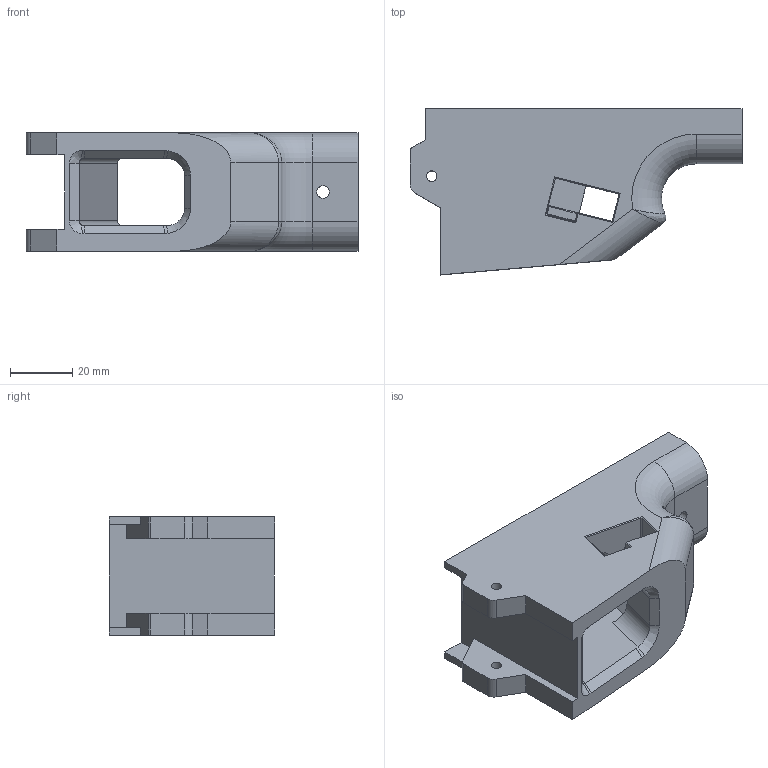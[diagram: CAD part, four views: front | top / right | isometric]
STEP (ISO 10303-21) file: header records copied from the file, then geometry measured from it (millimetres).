
FILE_DESCRIPTION(/* description */ (''),/* implementation_level */ '2;1');
FILE_NAME(/* author */ (''),/* organization */ (''),/* preprocessor_version */ 'ST-DEVELOPER v18.1',/* originating_system */ 'Autodesk Translation Framework v9.3.0.1241',/* authorisation */ '');
FILE_SCHEMA (('AUTOMOTIVE_DESIGN { 1 0 10303 214 3 1 1 }'));
Length unit declared in the file: inch
Products named in the file (1): beretta magwell practice
Bounding box: 106.5 x 53.2 x 38 mm (x, y, z)
Volume: 99738 mm3; surface area: 25918.8 mm2
Topology: 1 solids, 1 shells, 124 faces, 316 edges, 190 vertices
Faces by surface type: plane 85, cylinder 19, bspline 18, torus 2
Full cylindrical faces by diameter (mm): 3.401 x2, 4 x1
Entity records: 4115 total; most frequent: CARTESIAN_POINT 1203, ORIENTED_EDGE 628, DIRECTION 522, EDGE_CURVE 314, LINE 248, VECTOR 248, VERTEX_POINT 190, AXIS2_PLACEMENT_3D 137
